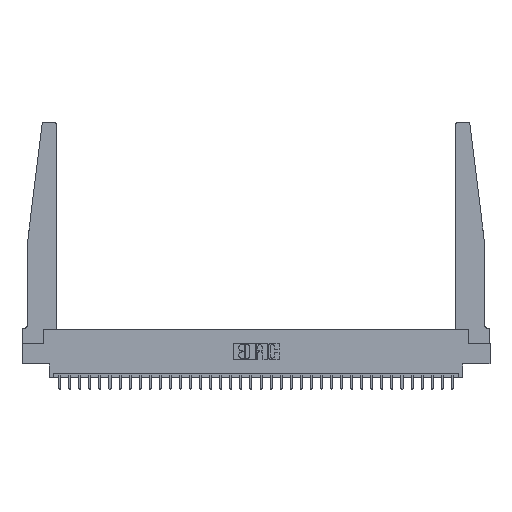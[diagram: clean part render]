
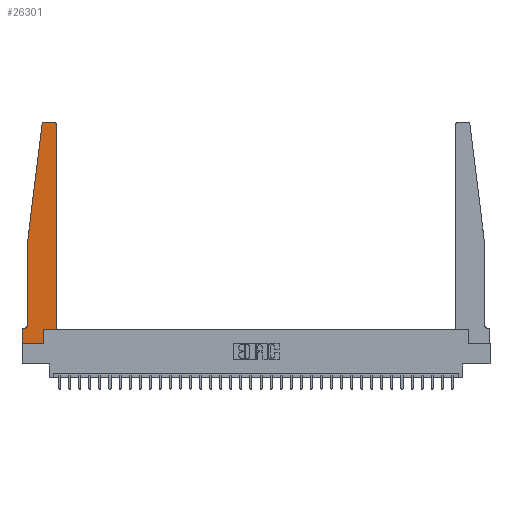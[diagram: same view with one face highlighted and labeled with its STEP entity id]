
A CAD part, top view. The second image highlights one B-rep face of the part: STEP entity #26301.
In plain terms, the highlighted planar face has unit normal (0, 0, 1).
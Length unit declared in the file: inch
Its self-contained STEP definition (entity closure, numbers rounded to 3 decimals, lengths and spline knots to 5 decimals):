
#186 = CARTESIAN_POINT ( 'NONE',  ( 0.425, 0.18, 0.37 ) ) ;
#296 = CIRCLE ( 'NONE', #5711, 0.03 ) ;
#589 = LINE ( 'NONE', #186, #25551 ) ;
#1144 = VECTOR ( 'NONE', #26683, 39.37008 ) ;
#1168 = VECTOR ( 'NONE', #18481, 39.37008 ) ;
#1485 = EDGE_CURVE ( 'NONE', #7830, #29905, #14132, .T. ) ;
#1987 = PLANE ( 'NONE',  #10669 ) ;
#2101 = CARTESIAN_POINT ( 'NONE',  ( 0.015, 0.2375, 0.37 ) ) ;
#2530 = VERTEX_POINT ( 'NONE', #25573 ) ;
#2644 = CARTESIAN_POINT ( 'NONE',  ( 0.2605, 0.18, 0.37 ) ) ;
#3935 = CARTESIAN_POINT ( 'NONE',  ( 0.425, 0.18, 0.37 ) ) ;
#4305 = CARTESIAN_POINT ( 'NONE',  ( 0.27653, 2.75, 0.37 ) ) ;
#4440 = DIRECTION ( 'NONE',  ( 1., 0., 0. ) ) ;
#4558 = DIRECTION ( 'NONE',  ( -1., 0., 0. ) ) ;
#5058 = CARTESIAN_POINT ( 'NONE',  ( 0.27653, 2.72, 0.37 ) ) ;
#5711 = AXIS2_PLACEMENT_3D ( 'NONE', #28581, #14260, #30999 ) ;
#5752 = EDGE_CURVE ( 'NONE', #8104, #7830, #14728, .T. ) ;
#5991 = DIRECTION ( 'NONE',  ( 0., 1., 0. ) ) ;
#6165 = ORIENTED_EDGE ( 'NONE', *, *, #7382, .T. ) ;
#6266 = ORIENTED_EDGE ( 'NONE', *, *, #15518, .T. ) ;
#6267 = LINE ( 'NONE', #14694, #31090 ) ;
#6615 = ORIENTED_EDGE ( 'NONE', *, *, #7527, .T. ) ;
#6682 = FACE_OUTER_BOUND ( 'NONE', #13504, .T. ) ;
#6879 = ORIENTED_EDGE ( 'NONE', *, *, #30598, .T. ) ;
#6929 = ORIENTED_EDGE ( 'NONE', *, *, #16618, .T. ) ;
#7059 = ORIENTED_EDGE ( 'NONE', *, *, #22534, .T. ) ;
#7109 = CARTESIAN_POINT ( 'NONE',  ( 0.2605, 0., 0.37 ) ) ;
#7119 = CARTESIAN_POINT ( 'NONE',  ( 0., 0.1875, 0.37 ) ) ;
#7330 = ORIENTED_EDGE ( 'NONE', *, *, #5752, .T. ) ;
#7369 = ORIENTED_EDGE ( 'NONE', *, *, #1485, .T. ) ;
#7382 = EDGE_CURVE ( 'NONE', #27672, #24855, #10075, .T. ) ;
#7421 = ORIENTED_EDGE ( 'NONE', *, *, #26050, .T. ) ;
#7504 = DIRECTION ( 'NONE',  ( 1., 0., 0. ) ) ;
#7527 = EDGE_CURVE ( 'NONE', #19648, #29822, #6267, .T. ) ;
#7543 = ORIENTED_EDGE ( 'NONE', *, *, #25088, .T. ) ;
#7784 = ORIENTED_EDGE ( 'NONE', *, *, #29111, .T. ) ;
#7830 = VERTEX_POINT ( 'NONE', #8508 ) ;
#8104 = VERTEX_POINT ( 'NONE', #7119 ) ;
#8423 = ORIENTED_EDGE ( 'NONE', *, *, #23511, .T. ) ;
#8508 = CARTESIAN_POINT ( 'NONE',  ( 0., 0., 0.37 ) ) ;
#8561 = LINE ( 'NONE', #27263, #13529 ) ;
#9411 = AXIS2_PLACEMENT_3D ( 'NONE', #5058, #21996, #7504 ) ;
#10073 = DIRECTION ( 'NONE',  ( 1., 0., 0. ) ) ;
#10075 = LINE ( 'NONE', #21427, #22886 ) ;
#10415 = CARTESIAN_POINT ( 'NONE',  ( 0.065, 0.1875, 0.37 ) ) ;
#10669 = AXIS2_PLACEMENT_3D ( 'NONE', #26037, #18986, #4440 ) ;
#11582 = VECTOR ( 'NONE', #12872, 39.37008 ) ;
#12356 = LINE ( 'NONE', #10415, #11582 ) ;
#12384 = CARTESIAN_POINT ( 'NONE',  ( 0., 0., 0.37 ) ) ;
#12872 = DIRECTION ( 'NONE',  ( -1., 0., 0. ) ) ;
#13504 = EDGE_LOOP ( 'NONE', ( #6165, #6266, #6615, #6879, #6929, #7059, #7330, #7369, #7421, #7543, #7784, #8423 ) ) ;
#13528 = VERTEX_POINT ( 'NONE', #17848 ) ;
#13529 = VECTOR ( 'NONE', #29685, 39.37008 ) ;
#14028 = CARTESIAN_POINT ( 'NONE',  ( 0.065, 1.25, 0.37 ) ) ;
#14132 = LINE ( 'NONE', #12384, #1144 ) ;
#14260 = DIRECTION ( 'NONE',  ( 0., 0., 1. ) ) ;
#14694 = CARTESIAN_POINT ( 'NONE',  ( 0.065, 1.25, 0.37 ) ) ;
#14728 = LINE ( 'NONE', #25214, #26675 ) ;
#15359 = CARTESIAN_POINT ( 'NONE',  ( 0.24675, 2.72367, 0.37 ) ) ;
#15518 = EDGE_CURVE ( 'NONE', #24855, #19648, #17586, .T. ) ;
#16618 = EDGE_CURVE ( 'NONE', #2530, #27591, #17961, .T. ) ;
#17586 = CIRCLE ( 'NONE', #9411, 0.03 ) ;
#17848 = CARTESIAN_POINT ( 'NONE',  ( 0.425, 2.72, 0.37 ) ) ;
#17961 = CIRCLE ( 'NONE', #25316, 0.05 ) ;
#18481 = DIRECTION ( 'NONE',  ( 0., 1., 0. ) ) ;
#18986 = DIRECTION ( 'NONE',  ( 0., 0., 1. ) ) ;
#19096 = DIRECTION ( 'NONE',  ( 0., 0., -1. ) ) ;
#19193 = LINE ( 'NONE', #20468, #27774 ) ;
#19585 = CARTESIAN_POINT ( 'NONE',  ( 0.425, 0.18, 0.37 ) ) ;
#19648 = VERTEX_POINT ( 'NONE', #15359 ) ;
#20468 = CARTESIAN_POINT ( 'NONE',  ( 0.2605, 0.18, 0.37 ) ) ;
#21427 = CARTESIAN_POINT ( 'NONE',  ( 0.25, 2.75, 0.37 ) ) ;
#21996 = DIRECTION ( 'NONE',  ( 0., 0., 1. ) ) ;
#22534 = EDGE_CURVE ( 'NONE', #27591, #8104, #12356, .T. ) ;
#22734 = CARTESIAN_POINT ( 'NONE',  ( 0.395, 2.75, 0.37 ) ) ;
#22868 = DIRECTION ( 'NONE',  ( 0., -1., 0. ) ) ;
#22886 = VECTOR ( 'NONE', #26176, 39.37008 ) ;
#23511 = EDGE_CURVE ( 'NONE', #13528, #27672, #296, .T. ) ;
#24855 = VERTEX_POINT ( 'NONE', #4305 ) ;
#25070 = VERTEX_POINT ( 'NONE', #19585 ) ;
#25088 = EDGE_CURVE ( 'NONE', #27466, #25070, #589, .T. ) ;
#25214 = CARTESIAN_POINT ( 'NONE',  ( 0., 0., 0.37 ) ) ;
#25316 = AXIS2_PLACEMENT_3D ( 'NONE', #2101, #19096, #4558 ) ;
#25551 = VECTOR ( 'NONE', #10073, 39.37008 ) ;
#25573 = CARTESIAN_POINT ( 'NONE',  ( 0.065, 0.2375, 0.37 ) ) ;
#26037 = CARTESIAN_POINT ( 'NONE',  ( 0., 0.1875, 0.37 ) ) ;
#26050 = EDGE_CURVE ( 'NONE', #29905, #27466, #19193, .T. ) ;
#26176 = DIRECTION ( 'NONE',  ( -1., 0., 0. ) ) ;
#26301 = ADVANCED_FACE ( 'NONE', ( #6682 ), #1987, .T. ) ;
#26588 = DIRECTION ( 'NONE',  ( -0.122, -0.992, 0. ) ) ;
#26675 = VECTOR ( 'NONE', #22868, 39.37008 ) ;
#26683 = DIRECTION ( 'NONE',  ( 1., 0., 0. ) ) ;
#26857 = LINE ( 'NONE', #3935, #1168 ) ;
#27263 = CARTESIAN_POINT ( 'NONE',  ( 0.065, 1.25, 0.37 ) ) ;
#27466 = VERTEX_POINT ( 'NONE', #2644 ) ;
#27591 = VERTEX_POINT ( 'NONE', #29744 ) ;
#27672 = VERTEX_POINT ( 'NONE', #22734 ) ;
#27774 = VECTOR ( 'NONE', #5991, 39.37008 ) ;
#28581 = CARTESIAN_POINT ( 'NONE',  ( 0.395, 2.72, 0.37 ) ) ;
#29111 = EDGE_CURVE ( 'NONE', #25070, #13528, #26857, .T. ) ;
#29685 = DIRECTION ( 'NONE',  ( 0., -1., 0. ) ) ;
#29744 = CARTESIAN_POINT ( 'NONE',  ( 0.015, 0.1875, 0.37 ) ) ;
#29822 = VERTEX_POINT ( 'NONE', #14028 ) ;
#29905 = VERTEX_POINT ( 'NONE', #7109 ) ;
#30598 = EDGE_CURVE ( 'NONE', #29822, #2530, #8561, .T. ) ;
#30999 = DIRECTION ( 'NONE',  ( 1., 0., 0. ) ) ;
#31090 = VECTOR ( 'NONE', #26588, 39.37008 ) ;
